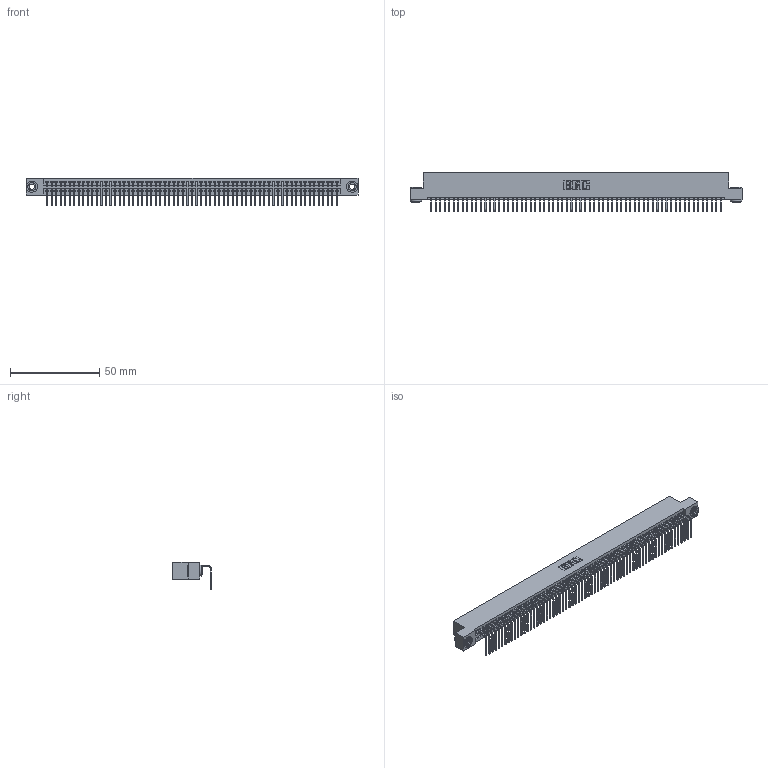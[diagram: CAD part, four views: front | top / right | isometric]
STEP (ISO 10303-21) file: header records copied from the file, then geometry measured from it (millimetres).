
FILE_DESCRIPTION (( 'STEP AP203' ), '1' );
FILE_NAME ('395-065-558-103.STEP', '2019-10-11T18:16:25', ( '' ), ( '' ), 'SwSTEP 2.0', 'SolidWorks 2016', '' );
FILE_SCHEMA (( 'CONFIG_CONTROL_DESIGN' ));
Length unit declared in the file: inch
Products named in the file (4): 395-065-558-103; 345 Part_Flush Mounting Lugs - 0.156 Dia-TH; 345-292-001_558 Tail - 2; 345-250-002_345-250-002-102
Assembly tree (68 placements, depth 2):
  395-065-558-103
    345 Part_Flush Mounting Lugs - 0.156 Dia-TH
    345-292-001_558 Tail - 2  x65
    345-250-002_345-250-002-102  x2
Bounding box: 186.31 x 21.83 x 15.37 mm (x, y, z)
Volume: 18120.2 mm3; surface area: 25879.7 mm2
Topology: 68 solids, 68 shells, 4064 faces, 12247 edges, 8074 vertices
Faces by surface type: plane 2820, cylinder 1236, cone 8
Entity records: 46558 total; most frequent: CARTESIAN_POINT 8042, ORIENTED_EDGE 8034, DIRECTION 7021, EDGE_CURVE 4017, VECTOR 3601, LINE 3601, VERTEX_POINT 2674, AXIS2_PLACEMENT_3D 1710
